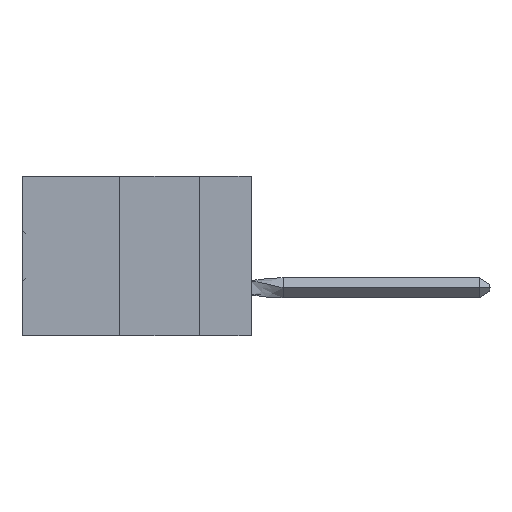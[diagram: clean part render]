
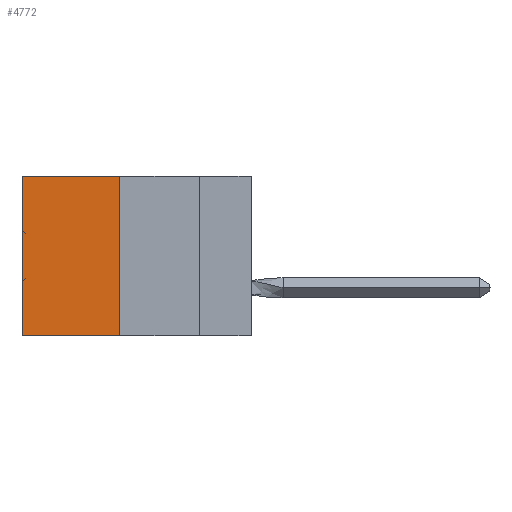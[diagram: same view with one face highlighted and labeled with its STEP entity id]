
A CAD part, left-side view. The second image highlights one B-rep face of the part: STEP entity #4772.
In plain terms, the highlighted planar face has unit normal (-1, 0, 0).
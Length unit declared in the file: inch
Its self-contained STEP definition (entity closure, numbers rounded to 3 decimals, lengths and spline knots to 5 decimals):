
#4772 = ADVANCED_FACE ( 'NONE', ( #6034 ), #36344, .F. ) ;
#4962 = VECTOR ( 'NONE', #14069, 39.37008 ) ;
#4998 = VECTOR ( 'NONE', #16969, 39.37008 ) ;
#6034 = FACE_OUTER_BOUND ( 'NONE', #58129, .T. ) ;
#7884 = CARTESIAN_POINT ( 'NONE',  ( 0.305, 0.72, -0.5 ) ) ;
#8085 = DIRECTION ( 'NONE',  ( 0., 0., -1. ) ) ;
#9124 = EDGE_CURVE ( 'NONE', #47806, #35293, #21982, .T. ) ;
#9687 = VERTEX_POINT ( 'NONE', #53529 ) ;
#10010 = LINE ( 'NONE', #21600, #4998 ) ;
#13260 = VECTOR ( 'NONE', #8085, 39.37008 ) ;
#14069 = DIRECTION ( 'NONE',  ( 0., 1., 0. ) ) ;
#14732 = LINE ( 'NONE', #7884, #13260 ) ;
#16969 = DIRECTION ( 'NONE',  ( 0., 0., -1. ) ) ;
#20546 = VECTOR ( 'NONE', #20909, 39.37008 ) ;
#20909 = DIRECTION ( 'NONE',  ( 0., 1., 0. ) ) ;
#21600 = CARTESIAN_POINT ( 'NONE',  ( 0.305, 0.413, -0.5 ) ) ;
#21861 = CARTESIAN_POINT ( 'NONE',  ( 0.305, 0.413, 0. ) ) ;
#21982 = LINE ( 'NONE', #29976, #20546 ) ;
#22650 = DIRECTION ( 'NONE',  ( 0., 0., -1. ) ) ;
#24121 = ORIENTED_EDGE ( 'NONE', *, *, #29882, .F. ) ;
#25508 = ORIENTED_EDGE ( 'NONE', *, *, #46144, .T. ) ;
#25842 = LINE ( 'NONE', #32949, #4962 ) ;
#29882 = EDGE_CURVE ( 'NONE', #49757, #47806, #10010, .T. ) ;
#29976 = CARTESIAN_POINT ( 'NONE',  ( 0.305, 0.413, -0.5 ) ) ;
#32949 = CARTESIAN_POINT ( 'NONE',  ( 0.305, 0.413, 0. ) ) ;
#35293 = VERTEX_POINT ( 'NONE', #54143 ) ;
#36344 = PLANE ( 'NONE',  #45408 ) ;
#36644 = EDGE_CURVE ( 'NONE', #49757, #9687, #25842, .T. ) ;
#38050 = ORIENTED_EDGE ( 'NONE', *, *, #9124, .F. ) ;
#39118 = ORIENTED_EDGE ( 'NONE', *, *, #36644, .T. ) ;
#41136 = DIRECTION ( 'NONE',  ( 1., 0., 0. ) ) ;
#44853 = CARTESIAN_POINT ( 'NONE',  ( 0.305, 0.413, -0.5 ) ) ;
#45408 = AXIS2_PLACEMENT_3D ( 'NONE', #45605, #41136, #22650 ) ;
#45605 = CARTESIAN_POINT ( 'NONE',  ( 0.305, 0.413, -0.5 ) ) ;
#46144 = EDGE_CURVE ( 'NONE', #9687, #35293, #14732, .T. ) ;
#47806 = VERTEX_POINT ( 'NONE', #44853 ) ;
#49757 = VERTEX_POINT ( 'NONE', #21861 ) ;
#53529 = CARTESIAN_POINT ( 'NONE',  ( 0.305, 0.72, 0. ) ) ;
#54143 = CARTESIAN_POINT ( 'NONE',  ( 0.305, 0.72, -0.5 ) ) ;
#58129 = EDGE_LOOP ( 'NONE', ( #25508, #38050, #24121, #39118 ) ) ;
